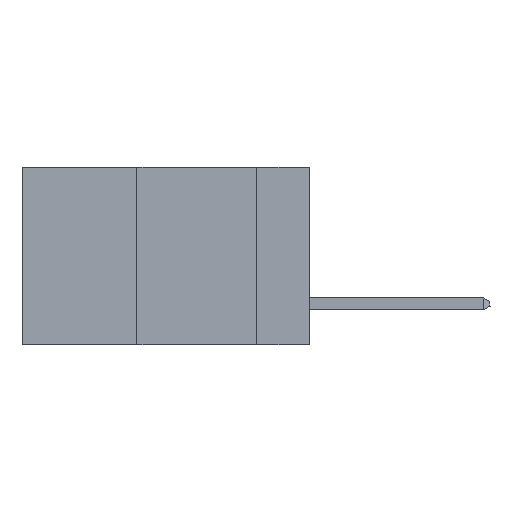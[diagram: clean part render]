
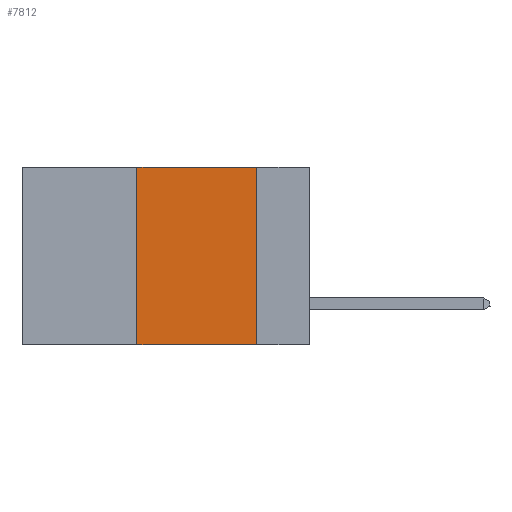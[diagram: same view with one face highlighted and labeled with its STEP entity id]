
A CAD part, left-side view. The second image highlights one B-rep face of the part: STEP entity #7812.
In plain terms, the highlighted planar face has unit normal (-1, 0, 0).
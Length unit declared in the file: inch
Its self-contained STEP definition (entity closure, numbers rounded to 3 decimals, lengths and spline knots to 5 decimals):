
#207 = VERTEX_POINT ( 'NONE', #8831 ) ;
#1481 = EDGE_CURVE ( 'NONE', #207, #10168, #4820, .T. ) ;
#1923 = CARTESIAN_POINT ( 'NONE',  ( 0., 0.11, 0. ) ) ;
#2340 = DIRECTION ( 'NONE',  ( 0., 0., -1. ) ) ;
#2643 = DIRECTION ( 'NONE',  ( 1., 0., 0. ) ) ;
#3138 = DIRECTION ( 'NONE',  ( 0., 0., 1. ) ) ;
#3479 = CARTESIAN_POINT ( 'NONE',  ( 0., 0.11, 0. ) ) ;
#3661 = EDGE_LOOP ( 'NONE', ( #11598, #6142, #11845, #7135 ) ) ;
#3864 = FACE_OUTER_BOUND ( 'NONE', #3661, .T. ) ;
#4229 = VERTEX_POINT ( 'NONE', #1923 ) ;
#4636 = VECTOR ( 'NONE', #8551, 39.37008 ) ;
#4820 = LINE ( 'NONE', #6227, #5270 ) ;
#5270 = VECTOR ( 'NONE', #3138, 39.37008 ) ;
#6142 = ORIENTED_EDGE ( 'NONE', *, *, #8853, .F. ) ;
#6227 = CARTESIAN_POINT ( 'NONE',  ( 0., 0.36, 0. ) ) ;
#7135 = ORIENTED_EDGE ( 'NONE', *, *, #10770, .T. ) ;
#7812 = ADVANCED_FACE ( 'NONE', ( #3864 ), #13743, .F. ) ;
#8551 = DIRECTION ( 'NONE',  ( 0., -1., 0. ) ) ;
#8831 = CARTESIAN_POINT ( 'NONE',  ( 0., 0.36, -0.37 ) ) ;
#8853 = EDGE_CURVE ( 'NONE', #10168, #4229, #9598, .T. ) ;
#9319 = CARTESIAN_POINT ( 'NONE',  ( 0., 0.6, 0. ) ) ;
#9380 = AXIS2_PLACEMENT_3D ( 'NONE', #15246, #2643, #12514 ) ;
#9598 = LINE ( 'NONE', #9319, #13930 ) ;
#9854 = CARTESIAN_POINT ( 'NONE',  ( 0., 0.6, -0.37 ) ) ;
#10168 = VERTEX_POINT ( 'NONE', #10739 ) ;
#10563 = VERTEX_POINT ( 'NONE', #12238 ) ;
#10649 = DIRECTION ( 'NONE',  ( 0., -1., 0. ) ) ;
#10739 = CARTESIAN_POINT ( 'NONE',  ( 0., 0.36, 0. ) ) ;
#10770 = EDGE_CURVE ( 'NONE', #207, #10563, #15520, .T. ) ;
#10950 = EDGE_CURVE ( 'NONE', #4229, #10563, #15220, .T. ) ;
#11598 = ORIENTED_EDGE ( 'NONE', *, *, #10950, .F. ) ;
#11845 = ORIENTED_EDGE ( 'NONE', *, *, #1481, .F. ) ;
#12238 = CARTESIAN_POINT ( 'NONE',  ( 0., 0.11, -0.37 ) ) ;
#12514 = DIRECTION ( 'NONE',  ( 0., 0., -1. ) ) ;
#13743 = PLANE ( 'NONE',  #9380 ) ;
#13930 = VECTOR ( 'NONE', #10649, 39.37008 ) ;
#14529 = VECTOR ( 'NONE', #2340, 39.37008 ) ;
#15220 = LINE ( 'NONE', #3479, #14529 ) ;
#15246 = CARTESIAN_POINT ( 'NONE',  ( 0., 0.6, 0. ) ) ;
#15520 = LINE ( 'NONE', #9854, #4636 ) ;
